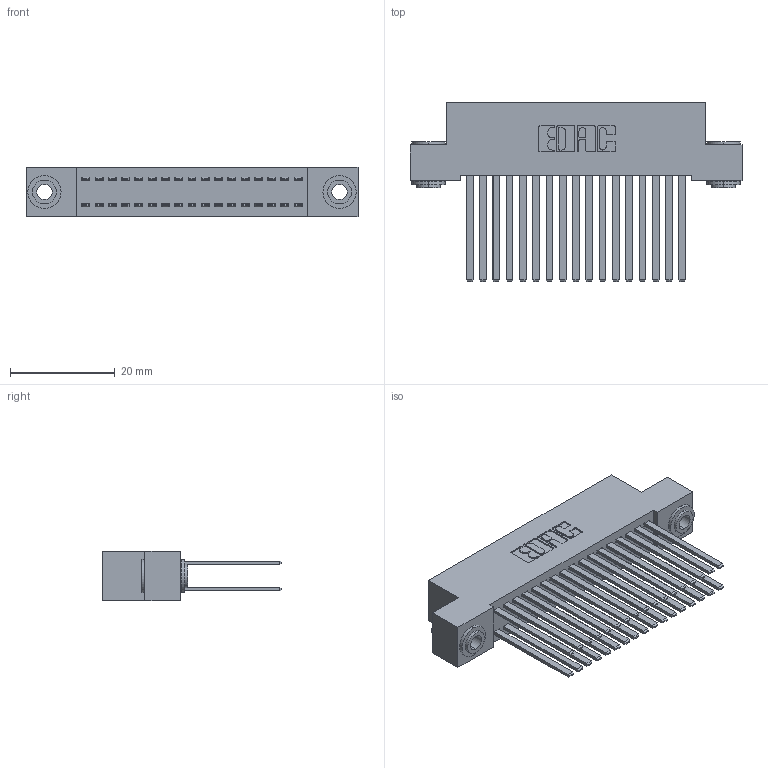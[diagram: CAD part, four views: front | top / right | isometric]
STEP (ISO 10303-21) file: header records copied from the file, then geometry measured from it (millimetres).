
FILE_DESCRIPTION (( 'STEP AP203' ), '1' );
FILE_NAME ('342-034-544-203.STEP', '2019-10-02T12:24:52', ( '' ), ( '' ), 'SwSTEP 2.0', 'SolidWorks 2016', '' );
FILE_SCHEMA (( 'CONFIG_CONTROL_DESIGN' ));
Length unit declared in the file: inch
Products named in the file (4): 342 Part_.156 TH; 345-292-001_345-293-144; 342-250-002_345-250-002-102; 342-034-544-203
Assembly tree (37 placements, depth 2):
  342-034-544-203
    342 Part_.156 TH
    345-292-001_345-293-144  x34
    342-250-002_345-250-002-102  x2
Bounding box: 63.5 x 34.3 x 9.4 mm (x, y, z)
Volume: 6086.6 mm3; surface area: 10825.4 mm2
Topology: 37 solids, 37 shells, 1712 faces, 5033 edges, 3306 vertices
Faces by surface type: plane 1164, cylinder 540, cone 8
Entity records: 14504 total; most frequent: CARTESIAN_POINT 2405, ORIENTED_EDGE 2334, DIRECTION 2129, EDGE_CURVE 1167, LINE 1019, VECTOR 1019, VERTEX_POINT 774, AXIS2_PLACEMENT_3D 555
